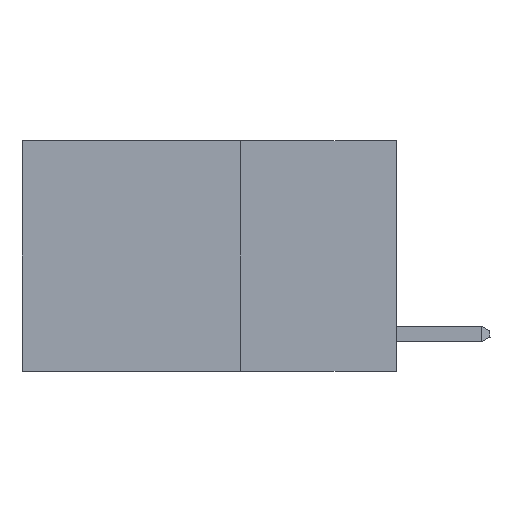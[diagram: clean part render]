
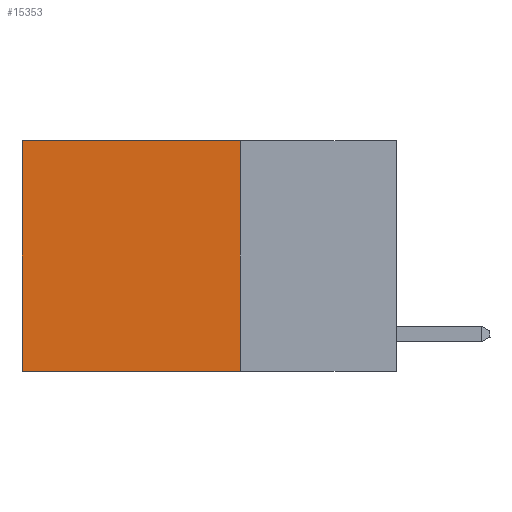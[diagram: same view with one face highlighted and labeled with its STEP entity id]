
A CAD part, left-side view. The second image highlights one B-rep face of the part: STEP entity #15353.
In plain terms, the highlighted planar face has unit normal (-1, 0, 0).
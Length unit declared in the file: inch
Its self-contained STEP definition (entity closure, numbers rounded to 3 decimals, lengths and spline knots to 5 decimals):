
#962 = DIRECTION ( 'NONE',  ( 1., 0., 0. ) ) ;
#1544 = CARTESIAN_POINT ( 'NONE',  ( 0.2625, 0.25, 0. ) ) ;
#1652 = VERTEX_POINT ( 'NONE', #15291 ) ;
#2456 = VECTOR ( 'NONE', #19986, 39.37008 ) ;
#2691 = ORIENTED_EDGE ( 'NONE', *, *, #14458, .T. ) ;
#3885 = EDGE_CURVE ( 'NONE', #4904, #8993, #19888, .T. ) ;
#4657 = LINE ( 'NONE', #14397, #12634 ) ;
#4904 = VERTEX_POINT ( 'NONE', #20254 ) ;
#5755 = CARTESIAN_POINT ( 'NONE',  ( 0.2625, 0.6, -0.37 ) ) ;
#6761 = VERTEX_POINT ( 'NONE', #9622 ) ;
#8078 = DIRECTION ( 'NONE',  ( 0., 0., -1. ) ) ;
#8993 = VERTEX_POINT ( 'NONE', #5755 ) ;
#9219 = DIRECTION ( 'NONE',  ( 0., 0., -1. ) ) ;
#9280 = DIRECTION ( 'NONE',  ( 0., 1., 0. ) ) ;
#9380 = CARTESIAN_POINT ( 'NONE',  ( 0.2625, 0.25, -0.37 ) ) ;
#9484 = LINE ( 'NONE', #1544, #14190 ) ;
#9586 = EDGE_CURVE ( 'NONE', #1652, #6761, #9484, .T. ) ;
#9622 = CARTESIAN_POINT ( 'NONE',  ( 0.2625, 0.25, -0.37 ) ) ;
#10546 = AXIS2_PLACEMENT_3D ( 'NONE', #15528, #962, #9219 ) ;
#11729 = CARTESIAN_POINT ( 'NONE',  ( 0.2625, 0.6, 0. ) ) ;
#12634 = VECTOR ( 'NONE', #20816, 39.37008 ) ;
#13821 = VECTOR ( 'NONE', #9280, 39.37008 ) ;
#14190 = VECTOR ( 'NONE', #8078, 39.37008 ) ;
#14397 = CARTESIAN_POINT ( 'NONE',  ( 0.2625, 0.25, 0. ) ) ;
#14458 = EDGE_CURVE ( 'NONE', #1652, #4904, #4657, .T. ) ;
#14634 = ORIENTED_EDGE ( 'NONE', *, *, #9586, .F. ) ;
#15127 = EDGE_LOOP ( 'NONE', ( #15320, #18343, #14634, #2691 ) ) ;
#15291 = CARTESIAN_POINT ( 'NONE',  ( 0.2625, 0.25, 0. ) ) ;
#15320 = ORIENTED_EDGE ( 'NONE', *, *, #3885, .T. ) ;
#15353 = ADVANCED_FACE ( 'NONE', ( #15859 ), #15961, .F. ) ;
#15528 = CARTESIAN_POINT ( 'NONE',  ( 0.2625, 0.25, 0. ) ) ;
#15768 = EDGE_CURVE ( 'NONE', #6761, #8993, #15909, .T. ) ;
#15859 = FACE_OUTER_BOUND ( 'NONE', #15127, .T. ) ;
#15909 = LINE ( 'NONE', #9380, #13821 ) ;
#15961 = PLANE ( 'NONE',  #10546 ) ;
#18343 = ORIENTED_EDGE ( 'NONE', *, *, #15768, .F. ) ;
#19888 = LINE ( 'NONE', #11729, #2456 ) ;
#19986 = DIRECTION ( 'NONE',  ( 0., 0., -1. ) ) ;
#20254 = CARTESIAN_POINT ( 'NONE',  ( 0.2625, 0.6, 0. ) ) ;
#20816 = DIRECTION ( 'NONE',  ( 0., 1., 0. ) ) ;
